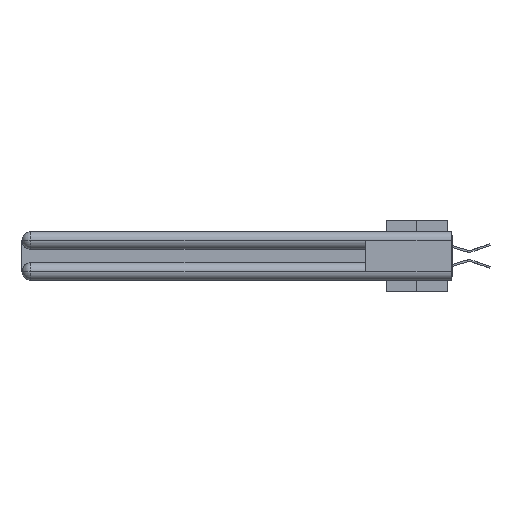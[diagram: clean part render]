
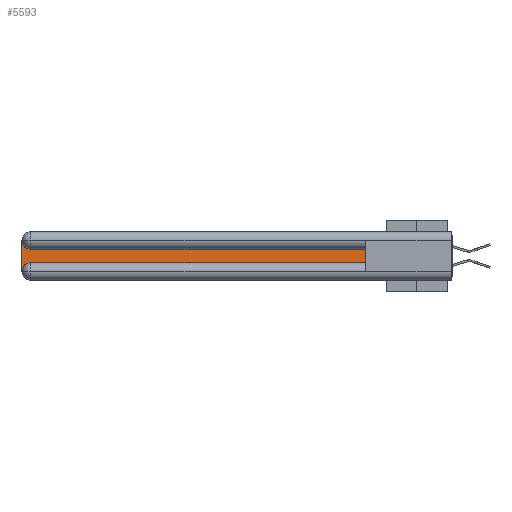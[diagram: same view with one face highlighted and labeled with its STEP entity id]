
A CAD part, left-side view. The second image highlights one B-rep face of the part: STEP entity #5593.
In plain terms, the highlighted planar face has unit normal (-1, 0, 0).
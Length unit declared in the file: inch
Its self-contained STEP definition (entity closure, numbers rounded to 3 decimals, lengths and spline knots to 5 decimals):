
#198 = DIRECTION ( 'NONE',  ( 1., 0., 0. ) ) ;
#751 = EDGE_CURVE ( 'NONE', #6182, #34496, #34862, .T. ) ;
#967 = LINE ( 'NONE', #36151, #38258 ) ;
#1160 = CARTESIAN_POINT ( 'NONE',  ( 0.075, 0.6, -0.2175 ) ) ;
#2043 = VERTEX_POINT ( 'NONE', #19404 ) ;
#2625 = CARTESIAN_POINT ( 'NONE',  ( 0.075, 0.6, -0.2175 ) ) ;
#2957 = CARTESIAN_POINT ( 'NONE',  ( 0.075, 2.94, -0.0625 ) ) ;
#4016 = AXIS2_PLACEMENT_3D ( 'NONE', #2957, #198, #29823 ) ;
#5593 = ADVANCED_FACE ( 'NONE', ( #33907 ), #7458, .F. ) ;
#5594 = CARTESIAN_POINT ( 'NONE',  ( 0.075, 0.6, -0.1225 ) ) ;
#6182 = VERTEX_POINT ( 'NONE', #9926 ) ;
#6397 = EDGE_CURVE ( 'NONE', #34496, #31458, #25301, .T. ) ;
#7458 = PLANE ( 'NONE',  #37491 ) ;
#7886 = DIRECTION ( 'NONE',  ( 0., 0., -1. ) ) ;
#9123 = DIRECTION ( 'NONE',  ( 0., -1., 0. ) ) ;
#9926 = CARTESIAN_POINT ( 'NONE',  ( 0.075, 2.94, -0.1225 ) ) ;
#10125 = ORIENTED_EDGE ( 'NONE', *, *, #6397, .T. ) ;
#10137 = CARTESIAN_POINT ( 'NONE',  ( 0.075, 3., -0.1225 ) ) ;
#10390 = DIRECTION ( 'NONE',  ( 0., 0., -1. ) ) ;
#11944 = CIRCLE ( 'NONE', #12541, 0.06 ) ;
#12541 = AXIS2_PLACEMENT_3D ( 'NONE', #20365, #35721, #29743 ) ;
#13461 = CARTESIAN_POINT ( 'NONE',  ( 0.075, 3., -0.0625 ) ) ;
#15935 = VECTOR ( 'NONE', #20346, 39.37008 ) ;
#16311 = DIRECTION ( 'NONE',  ( 0., 0., 1. ) ) ;
#19215 = LINE ( 'NONE', #1160, #21574 ) ;
#19404 = CARTESIAN_POINT ( 'NONE',  ( 0.075, 2.94, -0.2175 ) ) ;
#19984 = EDGE_LOOP ( 'NONE', ( #35532, #31249, #10125, #24448, #20995, #31407 ) ) ;
#20186 = EDGE_CURVE ( 'NONE', #2043, #29025, #967, .T. ) ;
#20346 = DIRECTION ( 'NONE',  ( 0., 1., 0. ) ) ;
#20365 = CARTESIAN_POINT ( 'NONE',  ( 0.075, 2.94, -0.2775 ) ) ;
#20995 = ORIENTED_EDGE ( 'NONE', *, *, #20186, .T. ) ;
#21055 = VECTOR ( 'NONE', #7886, 39.37008 ) ;
#21574 = VECTOR ( 'NONE', #16311, 39.37008 ) ;
#22737 = CARTESIAN_POINT ( 'NONE',  ( 0.075, 3., -0.2175 ) ) ;
#23969 = LINE ( 'NONE', #5594, #15935 ) ;
#24448 = ORIENTED_EDGE ( 'NONE', *, *, #24489, .T. ) ;
#24489 = EDGE_CURVE ( 'NONE', #31458, #2043, #11944, .T. ) ;
#25301 = LINE ( 'NONE', #22737, #21055 ) ;
#29025 = VERTEX_POINT ( 'NONE', #2625 ) ;
#29743 = DIRECTION ( 'NONE',  ( 0., 0., -1. ) ) ;
#29823 = DIRECTION ( 'NONE',  ( 0., 0., -1. ) ) ;
#31249 = ORIENTED_EDGE ( 'NONE', *, *, #751, .T. ) ;
#31407 = ORIENTED_EDGE ( 'NONE', *, *, #37893, .T. ) ;
#31458 = VERTEX_POINT ( 'NONE', #38402 ) ;
#31718 = CARTESIAN_POINT ( 'NONE',  ( 0.075, 0.6, -0.1225 ) ) ;
#33799 = EDGE_CURVE ( 'NONE', #34704, #6182, #23969, .T. ) ;
#33907 = FACE_OUTER_BOUND ( 'NONE', #19984, .T. ) ;
#34496 = VERTEX_POINT ( 'NONE', #13461 ) ;
#34704 = VERTEX_POINT ( 'NONE', #31718 ) ;
#34862 = CIRCLE ( 'NONE', #4016, 0.06 ) ;
#35532 = ORIENTED_EDGE ( 'NONE', *, *, #33799, .T. ) ;
#35721 = DIRECTION ( 'NONE',  ( 1., 0., 0. ) ) ;
#36151 = CARTESIAN_POINT ( 'NONE',  ( 0.075, 0.6, -0.2175 ) ) ;
#37290 = DIRECTION ( 'NONE',  ( 1., 0., 0. ) ) ;
#37491 = AXIS2_PLACEMENT_3D ( 'NONE', #10137, #37290, #10390 ) ;
#37893 = EDGE_CURVE ( 'NONE', #29025, #34704, #19215, .T. ) ;
#38258 = VECTOR ( 'NONE', #9123, 39.37008 ) ;
#38402 = CARTESIAN_POINT ( 'NONE',  ( 0.075, 3., -0.2775 ) ) ;
